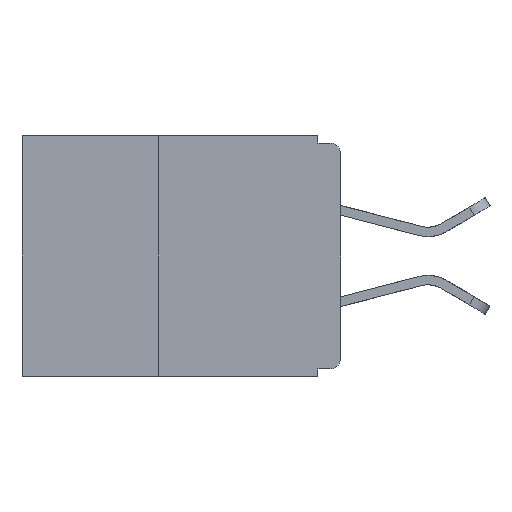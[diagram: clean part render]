
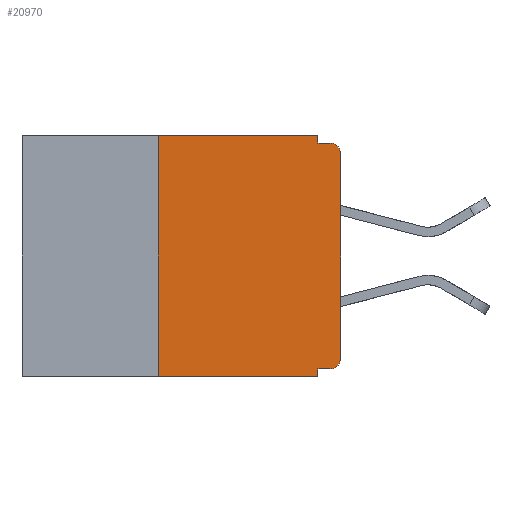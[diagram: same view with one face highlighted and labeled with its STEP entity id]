
A CAD part, left-side view. The second image highlights one B-rep face of the part: STEP entity #20970.
In plain terms, the highlighted planar face has unit normal (-1, 0, 0).
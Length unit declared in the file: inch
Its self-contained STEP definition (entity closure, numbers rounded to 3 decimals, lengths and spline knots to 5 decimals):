
#7 = FACE_OUTER_BOUND ( 'NONE', #13015, .T. ) ;
#164 = DIRECTION ( 'NONE',  ( 0., 0., -1. ) ) ;
#284 = EDGE_CURVE ( 'NONE', #2254, #2485, #767, .T. ) ;
#767 = LINE ( 'NONE', #8188, #14926 ) ;
#1007 = CARTESIAN_POINT ( 'NONE',  ( 0., 0.25, -0.33 ) ) ;
#1074 = ORIENTED_EDGE ( 'NONE', *, *, #13804, .F. ) ;
#1183 = CARTESIAN_POINT ( 'NONE',  ( 0., 0., 0. ) ) ;
#1429 = DIRECTION ( 'NONE',  ( 0., 0., -1. ) ) ;
#1830 = CARTESIAN_POINT ( 'NONE',  ( 0., 0.437, 0. ) ) ;
#1851 = CIRCLE ( 'NONE', #12189, 0.015 ) ;
#1928 = VERTEX_POINT ( 'NONE', #5456 ) ;
#2254 = VERTEX_POINT ( 'NONE', #8998 ) ;
#2337 = LINE ( 'NONE', #1007, #16475 ) ;
#2485 = VERTEX_POINT ( 'NONE', #8804 ) ;
#2760 = LINE ( 'NONE', #11043, #7263 ) ;
#3038 = VERTEX_POINT ( 'NONE', #19972 ) ;
#3490 = CARTESIAN_POINT ( 'NONE',  ( 0., 0.437, 0. ) ) ;
#3895 = CARTESIAN_POINT ( 'NONE',  ( 0., 0.015, -0.025 ) ) ;
#4226 = VERTEX_POINT ( 'NONE', #12784 ) ;
#4247 = EDGE_CURVE ( 'NONE', #6215, #1928, #19228, .T. ) ;
#4374 = LINE ( 'NONE', #19303, #13941 ) ;
#4778 = EDGE_CURVE ( 'NONE', #9867, #4226, #21282, .T. ) ;
#4878 = EDGE_CURVE ( 'NONE', #3038, #2254, #24492, .T. ) ;
#4967 = CARTESIAN_POINT ( 'NONE',  ( 0., 0.25, -0.33 ) ) ;
#5456 = CARTESIAN_POINT ( 'NONE',  ( 0., 0.031, 0. ) ) ;
#5805 = EDGE_CURVE ( 'NONE', #10629, #2485, #18271, .T. ) ;
#5815 = DIRECTION ( 'NONE',  ( 0., 0., -1. ) ) ;
#6215 = VERTEX_POINT ( 'NONE', #16900 ) ;
#6339 = ORIENTED_EDGE ( 'NONE', *, *, #22868, .F. ) ;
#6569 = EDGE_CURVE ( 'NONE', #3038, #9867, #7113, .T. ) ;
#7113 = CIRCLE ( 'NONE', #13802, 0.015 ) ;
#7263 = VECTOR ( 'NONE', #1429, 39.37008 ) ;
#7327 = DIRECTION ( 'NONE',  ( 0., 0., -1. ) ) ;
#7796 = ORIENTED_EDGE ( 'NONE', *, *, #4247, .F. ) ;
#7803 = ORIENTED_EDGE ( 'NONE', *, *, #11879, .F. ) ;
#8188 = CARTESIAN_POINT ( 'NONE',  ( 0., 0.031, -0.33 ) ) ;
#8470 = ORIENTED_EDGE ( 'NONE', *, *, #284, .F. ) ;
#8589 = DIRECTION ( 'NONE',  ( 0., 0., 1. ) ) ;
#8804 = CARTESIAN_POINT ( 'NONE',  ( 0., 0.031, -0.33 ) ) ;
#8998 = CARTESIAN_POINT ( 'NONE',  ( 0., 0.031, -0.32 ) ) ;
#9276 = ORIENTED_EDGE ( 'NONE', *, *, #4778, .T. ) ;
#9867 = VERTEX_POINT ( 'NONE', #16063 ) ;
#10629 = VERTEX_POINT ( 'NONE', #4967 ) ;
#11043 = CARTESIAN_POINT ( 'NONE',  ( 0., 0.031, 0. ) ) ;
#11125 = VECTOR ( 'NONE', #8589, 39.37008 ) ;
#11790 = ORIENTED_EDGE ( 'NONE', *, *, #19826, .T. ) ;
#11879 = EDGE_CURVE ( 'NONE', #1928, #12022, #2760, .T. ) ;
#12022 = VERTEX_POINT ( 'NONE', #19157 ) ;
#12028 = DIRECTION ( 'NONE',  ( 0., 0., -1. ) ) ;
#12056 = DIRECTION ( 'NONE',  ( -1., 0., 0. ) ) ;
#12080 = CARTESIAN_POINT ( 'NONE',  ( 0., 0.015, -0.305 ) ) ;
#12189 = AXIS2_PLACEMENT_3D ( 'NONE', #3895, #17314, #5815 ) ;
#12574 = DIRECTION ( 'NONE',  ( 0., 0., 1. ) ) ;
#12784 = CARTESIAN_POINT ( 'NONE',  ( 0., 0., -0.025 ) ) ;
#12790 = DIRECTION ( 'NONE',  ( 0., -1., 0. ) ) ;
#13015 = EDGE_LOOP ( 'NONE', ( #9276, #11790, #6339, #7803, #7796, #1074, #17605, #8470, #14920, #16076 ) ) ;
#13143 = VECTOR ( 'NONE', #23914, 39.37008 ) ;
#13802 = AXIS2_PLACEMENT_3D ( 'NONE', #12080, #12056, #12028 ) ;
#13804 = EDGE_CURVE ( 'NONE', #10629, #6215, #2337, .T. ) ;
#13941 = VECTOR ( 'NONE', #21215, 39.37008 ) ;
#14114 = AXIS2_PLACEMENT_3D ( 'NONE', #3490, #18808, #7327 ) ;
#14920 = ORIENTED_EDGE ( 'NONE', *, *, #4878, .F. ) ;
#14926 = VECTOR ( 'NONE', #164, 39.37008 ) ;
#16063 = CARTESIAN_POINT ( 'NONE',  ( 0., 0., -0.305 ) ) ;
#16076 = ORIENTED_EDGE ( 'NONE', *, *, #6569, .T. ) ;
#16475 = VECTOR ( 'NONE', #12574, 39.37008 ) ;
#16900 = CARTESIAN_POINT ( 'NONE',  ( 0., 0.25, 0. ) ) ;
#16913 = PLANE ( 'NONE',  #14114 ) ;
#17314 = DIRECTION ( 'NONE',  ( -1., 0., 0. ) ) ;
#17605 = ORIENTED_EDGE ( 'NONE', *, *, #5805, .T. ) ;
#18271 = LINE ( 'NONE', #24178, #13143 ) ;
#18638 = VECTOR ( 'NONE', #12790, 39.37008 ) ;
#18808 = DIRECTION ( 'NONE',  ( 1., 0., 0. ) ) ;
#19157 = CARTESIAN_POINT ( 'NONE',  ( 0., 0.031, -0.01 ) ) ;
#19228 = LINE ( 'NONE', #1830, #18638 ) ;
#19303 = CARTESIAN_POINT ( 'NONE',  ( 0., 0., -0.01 ) ) ;
#19344 = DIRECTION ( 'NONE',  ( 0., 1., 0. ) ) ;
#19826 = EDGE_CURVE ( 'NONE', #4226, #21625, #1851, .T. ) ;
#19972 = CARTESIAN_POINT ( 'NONE',  ( 0., 0.015, -0.32 ) ) ;
#20402 = CARTESIAN_POINT ( 'NONE',  ( 0., 0., -0.32 ) ) ;
#20970 = ADVANCED_FACE ( 'NONE', ( #7 ), #16913, .F. ) ;
#21110 = CARTESIAN_POINT ( 'NONE',  ( 0., 0.015, -0.01 ) ) ;
#21215 = DIRECTION ( 'NONE',  ( 0., -1., 0. ) ) ;
#21282 = LINE ( 'NONE', #1183, #11125 ) ;
#21625 = VERTEX_POINT ( 'NONE', #21110 ) ;
#22868 = EDGE_CURVE ( 'NONE', #12022, #21625, #4374, .T. ) ;
#23901 = VECTOR ( 'NONE', #19344, 39.37008 ) ;
#23914 = DIRECTION ( 'NONE',  ( 0., -1., 0. ) ) ;
#24178 = CARTESIAN_POINT ( 'NONE',  ( 0., 0.437, -0.33 ) ) ;
#24492 = LINE ( 'NONE', #20402, #23901 ) ;
